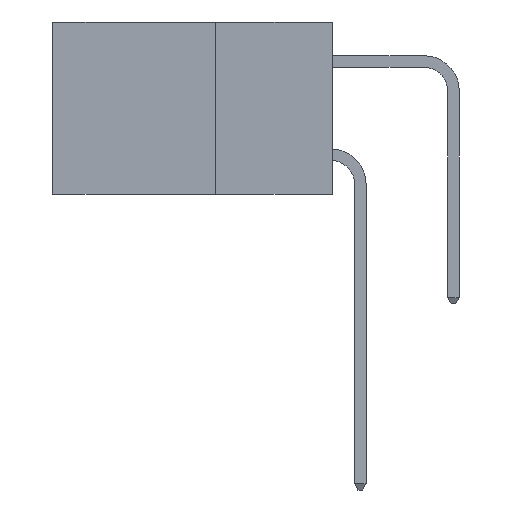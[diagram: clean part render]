
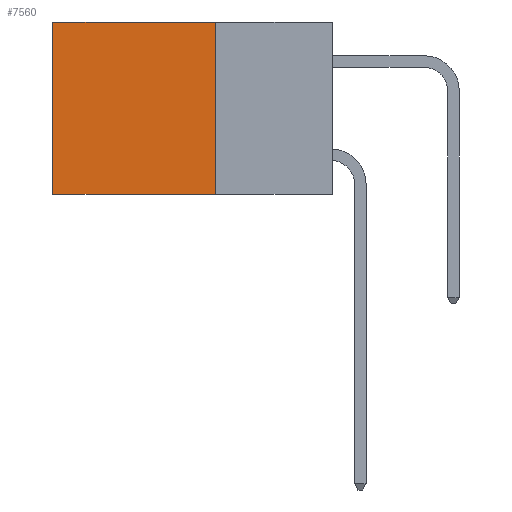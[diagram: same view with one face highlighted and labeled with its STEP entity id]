
A CAD part, left-side view. The second image highlights one B-rep face of the part: STEP entity #7560.
In plain terms, the highlighted planar face has unit normal (-1, 0, 0).
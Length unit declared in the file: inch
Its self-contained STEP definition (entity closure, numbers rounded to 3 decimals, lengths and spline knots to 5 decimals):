
#666 = VECTOR ( 'NONE', #19623, 39.37008 ) ;
#786 = DIRECTION ( 'NONE',  ( 0., 0., -1. ) ) ;
#977 = VECTOR ( 'NONE', #10803, 39.37008 ) ;
#1166 = LINE ( 'NONE', #11871, #666 ) ;
#1210 = AXIS2_PLACEMENT_3D ( 'NONE', #18486, #10585, #786 ) ;
#1518 = ORIENTED_EDGE ( 'NONE', *, *, #3863, .T. ) ;
#1789 = CARTESIAN_POINT ( 'NONE',  ( 0.2615, 0.6, 0. ) ) ;
#2865 = EDGE_CURVE ( 'NONE', #13223, #4431, #5572, .T. ) ;
#3863 = EDGE_CURVE ( 'NONE', #16468, #3921, #18162, .T. ) ;
#3921 = VERTEX_POINT ( 'NONE', #8190 ) ;
#3975 = DIRECTION ( 'NONE',  ( 0., 1., 0. ) ) ;
#4405 = ORIENTED_EDGE ( 'NONE', *, *, #7022, .T. ) ;
#4431 = VERTEX_POINT ( 'NONE', #8504 ) ;
#5572 = LINE ( 'NONE', #14672, #9450 ) ;
#7022 = EDGE_CURVE ( 'NONE', #13223, #16468, #19808, .T. ) ;
#7099 = VECTOR ( 'NONE', #3975, 39.37008 ) ;
#7259 = PLANE ( 'NONE',  #1210 ) ;
#7560 = ADVANCED_FACE ( 'NONE', ( #13294 ), #7259, .F. ) ;
#8190 = CARTESIAN_POINT ( 'NONE',  ( 0.2615, 0.6, -0.37 ) ) ;
#8191 = EDGE_CURVE ( 'NONE', #4431, #3921, #1166, .T. ) ;
#8368 = CARTESIAN_POINT ( 'NONE',  ( 0.2615, 0.25, 0. ) ) ;
#8504 = CARTESIAN_POINT ( 'NONE',  ( 0.2615, 0.25, -0.37 ) ) ;
#9450 = VECTOR ( 'NONE', #15859, 39.37008 ) ;
#10585 = DIRECTION ( 'NONE',  ( 1., 0., 0. ) ) ;
#10803 = DIRECTION ( 'NONE',  ( 0., 0., -1. ) ) ;
#10972 = CARTESIAN_POINT ( 'NONE',  ( 0.2615, 0.6, -0.37 ) ) ;
#11210 = ORIENTED_EDGE ( 'NONE', *, *, #8191, .F. ) ;
#11871 = CARTESIAN_POINT ( 'NONE',  ( 0.2615, 0.25, -0.37 ) ) ;
#13223 = VERTEX_POINT ( 'NONE', #8368 ) ;
#13294 = FACE_OUTER_BOUND ( 'NONE', #20217, .T. ) ;
#14235 = ORIENTED_EDGE ( 'NONE', *, *, #2865, .F. ) ;
#14672 = CARTESIAN_POINT ( 'NONE',  ( 0.2615, 0.25, -0.37 ) ) ;
#15859 = DIRECTION ( 'NONE',  ( 0., 0., -1. ) ) ;
#16468 = VERTEX_POINT ( 'NONE', #1789 ) ;
#18162 = LINE ( 'NONE', #10972, #977 ) ;
#18486 = CARTESIAN_POINT ( 'NONE',  ( 0.2615, 0.25, -0.37 ) ) ;
#19623 = DIRECTION ( 'NONE',  ( 0., 1., 0. ) ) ;
#19808 = LINE ( 'NONE', #20006, #7099 ) ;
#20006 = CARTESIAN_POINT ( 'NONE',  ( 0.2615, 0.25, 0. ) ) ;
#20217 = EDGE_LOOP ( 'NONE', ( #1518, #11210, #14235, #4405 ) ) ;
